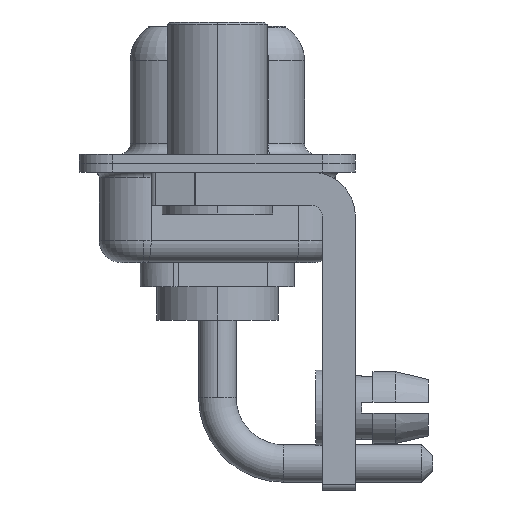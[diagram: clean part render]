
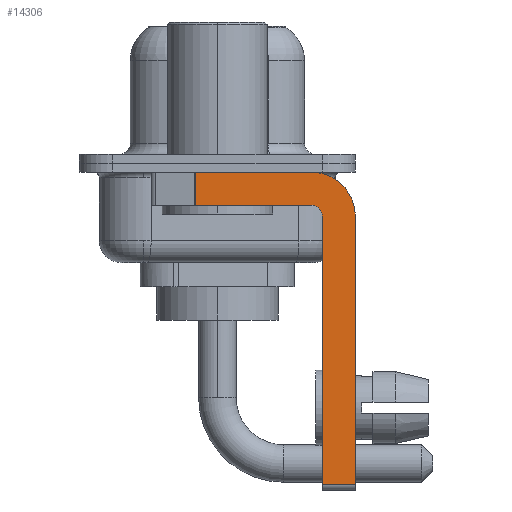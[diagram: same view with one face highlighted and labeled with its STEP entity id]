
A CAD part, left-side view. The second image highlights one B-rep face of the part: STEP entity #14306.
In plain terms, the highlighted planar face has unit normal (-1, 0, 0).
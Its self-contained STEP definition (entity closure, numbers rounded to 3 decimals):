
#269 = CIRCLE ( 'NONE', #11744, 2. ) ;
#441 = DIRECTION ( 'NONE',  ( 0., -1., 0. ) ) ;
#803 = CARTESIAN_POINT ( 'NONE',  ( -2.9, -6.25, -2.4 ) ) ;
#1194 = ORIENTED_EDGE ( 'NONE', *, *, #2279, .F. ) ;
#1226 = CARTESIAN_POINT ( 'NONE',  ( -2.9, -4.75, -14.8 ) ) ;
#1712 = DIRECTION ( 'NONE',  ( 0., 0., 1. ) ) ;
#1787 = CARTESIAN_POINT ( 'NONE',  ( -2.9, -4.25, -1.9 ) ) ;
#1990 = LINE ( 'NONE', #14659, #6824 ) ;
#2178 = CIRCLE ( 'NONE', #5859, 0.5 ) ;
#2273 = ORIENTED_EDGE ( 'NONE', *, *, #2831, .F. ) ;
#2279 = EDGE_CURVE ( 'NONE', #11716, #12876, #1990, .T. ) ;
#2308 = LINE ( 'NONE', #1226, #11666 ) ;
#2466 = EDGE_CURVE ( 'NONE', #7086, #15970, #2308, .T. ) ;
#2831 = EDGE_CURVE ( 'NONE', #14634, #5155, #4447, .T. ) ;
#3015 = DIRECTION ( 'NONE',  ( 0., 0., -1. ) ) ;
#3229 = DIRECTION ( 'NONE',  ( 0., 1., 0. ) ) ;
#3743 = VERTEX_POINT ( 'NONE', #6893 ) ;
#3932 = LINE ( 'NONE', #9031, #11531 ) ;
#4134 = FACE_OUTER_BOUND ( 'NONE', #12709, .T. ) ;
#4370 = DIRECTION ( 'NONE',  ( 0., -1., 0. ) ) ;
#4447 = LINE ( 'NONE', #8385, #10874 ) ;
#4732 = ORIENTED_EDGE ( 'NONE', *, *, #5985, .T. ) ;
#5155 = VERTEX_POINT ( 'NONE', #14813 ) ;
#5457 = EDGE_CURVE ( 'NONE', #15970, #11716, #2178, .T. ) ;
#5556 = PLANE ( 'NONE',  #14401 ) ;
#5859 = AXIS2_PLACEMENT_3D ( 'NONE', #6708, #13152, #1712 ) ;
#5985 = EDGE_CURVE ( 'NONE', #7086, #7009, #3932, .T. ) ;
#6198 = VECTOR ( 'NONE', #8567, 1000. ) ;
#6708 = CARTESIAN_POINT ( 'NONE',  ( -2.9, -4.25, -2.4 ) ) ;
#6824 = VECTOR ( 'NONE', #3229, 1000. ) ;
#6893 = CARTESIAN_POINT ( 'NONE',  ( -2.9, -6.25, -2.4 ) ) ;
#6926 = DIRECTION ( 'NONE',  ( 1., 0., 0. ) ) ;
#7009 = VERTEX_POINT ( 'NONE', #15976 ) ;
#7086 = VERTEX_POINT ( 'NONE', #16144 ) ;
#7590 = ORIENTED_EDGE ( 'NONE', *, *, #12078, .T. ) ;
#7819 = CARTESIAN_POINT ( 'NONE',  ( -2.9, -4.25, -2.4 ) ) ;
#8138 = EDGE_CURVE ( 'NONE', #3743, #7009, #14733, .T. ) ;
#8385 = CARTESIAN_POINT ( 'NONE',  ( -2.9, 3., -0.4 ) ) ;
#8567 = DIRECTION ( 'NONE',  ( 0., 0., -1. ) ) ;
#9031 = CARTESIAN_POINT ( 'NONE',  ( -2.9, -4.25, -14.55 ) ) ;
#10458 = CARTESIAN_POINT ( 'NONE',  ( -2.9, -4.25, -2.4 ) ) ;
#10538 = DIRECTION ( 'NONE',  ( 0., 0., -1. ) ) ;
#10669 = DIRECTION ( 'NONE',  ( 1., 0., 0. ) ) ;
#10874 = VECTOR ( 'NONE', #4370, 1000. ) ;
#10935 = VECTOR ( 'NONE', #3015, 1000. ) ;
#11131 = ORIENTED_EDGE ( 'NONE', *, *, #2466, .F. ) ;
#11531 = VECTOR ( 'NONE', #441, 1000. ) ;
#11558 = ORIENTED_EDGE ( 'NONE', *, *, #12108, .F. ) ;
#11666 = VECTOR ( 'NONE', #13747, 1000. ) ;
#11716 = VERTEX_POINT ( 'NONE', #1787 ) ;
#11744 = AXIS2_PLACEMENT_3D ( 'NONE', #10458, #6926, #10538 ) ;
#12078 = EDGE_CURVE ( 'NONE', #14634, #12876, #15537, .T. ) ;
#12102 = CARTESIAN_POINT ( 'NONE',  ( -2.9, 0.978, -0.4 ) ) ;
#12108 = EDGE_CURVE ( 'NONE', #5155, #3743, #269, .T. ) ;
#12709 = EDGE_LOOP ( 'NONE', ( #2273, #7590, #1194, #14182, #11131, #4732, #15113, #11558 ) ) ;
#12876 = VERTEX_POINT ( 'NONE', #16264 ) ;
#13152 = DIRECTION ( 'NONE',  ( -1., 0., 0. ) ) ;
#13609 = CARTESIAN_POINT ( 'NONE',  ( -2.9, -4.75, -2.4 ) ) ;
#13747 = DIRECTION ( 'NONE',  ( 0., 0., 1. ) ) ;
#14182 = ORIENTED_EDGE ( 'NONE', *, *, #5457, .F. ) ;
#14306 = ADVANCED_FACE ( 'NONE', ( #4134 ), #5556, .F. ) ;
#14401 = AXIS2_PLACEMENT_3D ( 'NONE', #7819, #10669, #15748 ) ;
#14612 = CARTESIAN_POINT ( 'NONE',  ( -2.9, 0.978, -1.9 ) ) ;
#14634 = VERTEX_POINT ( 'NONE', #12102 ) ;
#14659 = CARTESIAN_POINT ( 'NONE',  ( -2.9, -4.25, -1.9 ) ) ;
#14733 = LINE ( 'NONE', #803, #6198 ) ;
#14813 = CARTESIAN_POINT ( 'NONE',  ( -2.9, -4.25, -0.4 ) ) ;
#15113 = ORIENTED_EDGE ( 'NONE', *, *, #8138, .F. ) ;
#15537 = LINE ( 'NONE', #14612, #10935 ) ;
#15748 = DIRECTION ( 'NONE',  ( 0., 0., -1. ) ) ;
#15970 = VERTEX_POINT ( 'NONE', #13609 ) ;
#15976 = CARTESIAN_POINT ( 'NONE',  ( -2.9, -6.25, -14.55 ) ) ;
#16144 = CARTESIAN_POINT ( 'NONE',  ( -2.9, -4.75, -14.55 ) ) ;
#16264 = CARTESIAN_POINT ( 'NONE',  ( -2.9, 0.978, -1.9 ) ) ;
